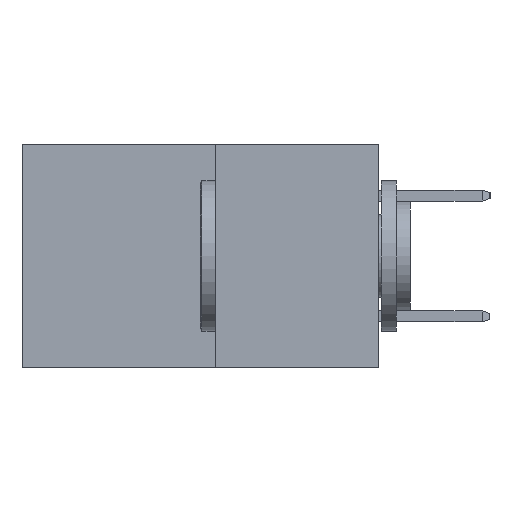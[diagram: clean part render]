
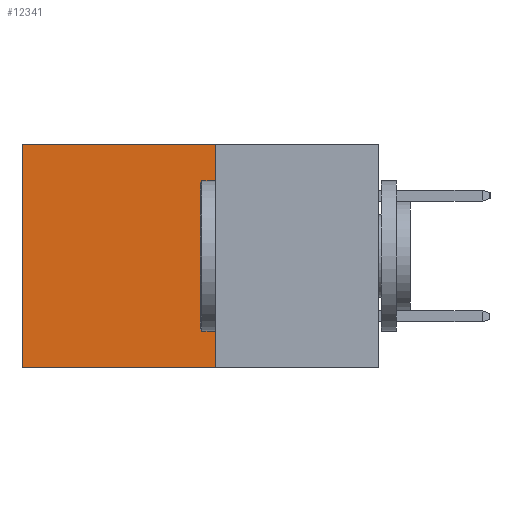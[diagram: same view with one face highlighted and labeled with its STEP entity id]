
A CAD part, left-side view. The second image highlights one B-rep face of the part: STEP entity #12341.
In plain terms, the highlighted planar face has unit normal (-1, 0, 0).
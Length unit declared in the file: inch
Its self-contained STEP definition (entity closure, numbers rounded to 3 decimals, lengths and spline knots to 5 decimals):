
#147 = VECTOR ( 'NONE', #4207, 39.37008 ) ;
#150 = EDGE_CURVE ( 'NONE', #6820, #12771, #11466, .T. ) ;
#763 = CARTESIAN_POINT ( 'NONE',  ( 0.277, 0.59, -0.37 ) ) ;
#1422 = CARTESIAN_POINT ( 'NONE',  ( 0.277, 0.27, 0. ) ) ;
#1829 = ORIENTED_EDGE ( 'NONE', *, *, #11263, .F. ) ;
#1906 = ORIENTED_EDGE ( 'NONE', *, *, #150, .F. ) ;
#2251 = DIRECTION ( 'NONE',  ( 1., 0., 0. ) ) ;
#2473 = ORIENTED_EDGE ( 'NONE', *, *, #11748, .T. ) ;
#2502 = VERTEX_POINT ( 'NONE', #1422 ) ;
#3921 = VERTEX_POINT ( 'NONE', #8380 ) ;
#4083 = CARTESIAN_POINT ( 'NONE',  ( 0.277, 0.27, -0.37 ) ) ;
#4207 = DIRECTION ( 'NONE',  ( 0., 1., 0. ) ) ;
#4429 = CARTESIAN_POINT ( 'NONE',  ( 0.277, 0.27, -0.37 ) ) ;
#5704 = EDGE_LOOP ( 'NONE', ( #2473, #1906, #1829, #7159 ) ) ;
#6571 = LINE ( 'NONE', #10991, #9049 ) ;
#6820 = VERTEX_POINT ( 'NONE', #7879 ) ;
#6830 = DIRECTION ( 'NONE',  ( 0., 0., -1. ) ) ;
#7159 = ORIENTED_EDGE ( 'NONE', *, *, #10843, .T. ) ;
#7856 = DIRECTION ( 'NONE',  ( 0., 1., 0. ) ) ;
#7879 = CARTESIAN_POINT ( 'NONE',  ( 0.277, 0.27, -0.37 ) ) ;
#8044 = LINE ( 'NONE', #13132, #13644 ) ;
#8380 = CARTESIAN_POINT ( 'NONE',  ( 0.277, 0.59, 0. ) ) ;
#8679 = PLANE ( 'NONE',  #10676 ) ;
#8689 = FACE_OUTER_BOUND ( 'NONE', #5704, .T. ) ;
#9049 = VECTOR ( 'NONE', #7856, 39.37008 ) ;
#9759 = DIRECTION ( 'NONE',  ( 0., 0., -1. ) ) ;
#9858 = CARTESIAN_POINT ( 'NONE',  ( 0.277, 0.59, -0.37 ) ) ;
#10489 = VECTOR ( 'NONE', #10897, 39.37008 ) ;
#10676 = AXIS2_PLACEMENT_3D ( 'NONE', #4429, #2251, #9759 ) ;
#10843 = EDGE_CURVE ( 'NONE', #2502, #3921, #6571, .T. ) ;
#10897 = DIRECTION ( 'NONE',  ( 0., 0., -1. ) ) ;
#10991 = CARTESIAN_POINT ( 'NONE',  ( 0.277, 0.27, 0. ) ) ;
#11263 = EDGE_CURVE ( 'NONE', #2502, #6820, #8044, .T. ) ;
#11466 = LINE ( 'NONE', #4083, #147 ) ;
#11748 = EDGE_CURVE ( 'NONE', #3921, #12771, #13302, .T. ) ;
#12341 = ADVANCED_FACE ( 'NONE', ( #8689 ), #8679, .F. ) ;
#12771 = VERTEX_POINT ( 'NONE', #763 ) ;
#13132 = CARTESIAN_POINT ( 'NONE',  ( 0.277, 0.27, -0.37 ) ) ;
#13302 = LINE ( 'NONE', #9858, #10489 ) ;
#13644 = VECTOR ( 'NONE', #6830, 39.37008 ) ;
